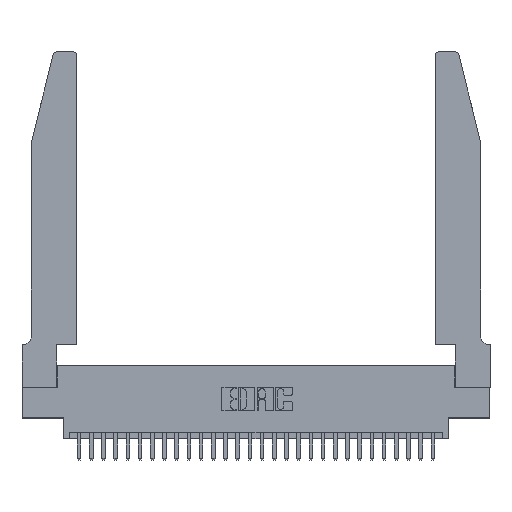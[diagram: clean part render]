
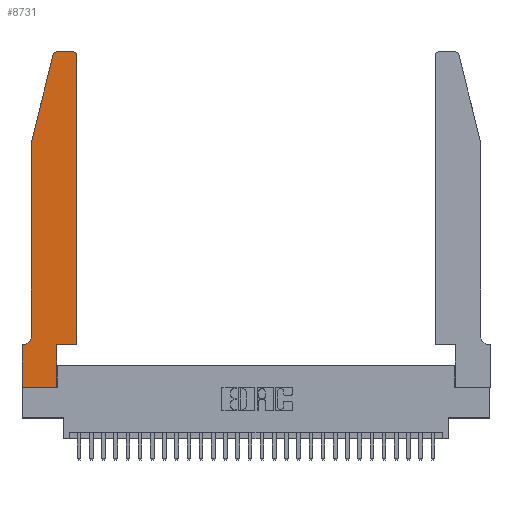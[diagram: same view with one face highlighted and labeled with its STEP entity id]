
A CAD part, top view. The second image highlights one B-rep face of the part: STEP entity #8731.
In plain terms, the highlighted planar face has unit normal (0, 0, 1).
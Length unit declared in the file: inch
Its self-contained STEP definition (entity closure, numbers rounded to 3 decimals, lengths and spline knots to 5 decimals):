
#400 = DIRECTION ( 'NONE',  ( 0., 1., 0. ) ) ;
#866 = VERTEX_POINT ( 'NONE', #1583 ) ;
#1382 = VERTEX_POINT ( 'NONE', #17906 ) ;
#1514 = CARTESIAN_POINT ( 'NONE',  ( 0.4505, 2.72, 0.37 ) ) ;
#1583 = CARTESIAN_POINT ( 'NONE',  ( 0., 0., 0.37 ) ) ;
#1839 = ORIENTED_EDGE ( 'NONE', *, *, #29687, .T. ) ;
#2173 = DIRECTION ( 'NONE',  ( -1., 0., 0. ) ) ;
#2347 = DIRECTION ( 'NONE',  ( 0., 0., 1. ) ) ;
#2519 = AXIS2_PLACEMENT_3D ( 'NONE', #6919, #2347, #13959 ) ;
#2740 = FACE_OUTER_BOUND ( 'NONE', #25307, .T. ) ;
#2749 = LINE ( 'NONE', #6839, #7132 ) ;
#3153 = DIRECTION ( 'NONE',  ( 1., 0., 0. ) ) ;
#3450 = VECTOR ( 'NONE', #23877, 39.37008 ) ;
#3625 = CARTESIAN_POINT ( 'NONE',  ( 0.0055, 0.42, 0.37 ) ) ;
#4006 = ORIENTED_EDGE ( 'NONE', *, *, #6376, .T. ) ;
#4008 = CARTESIAN_POINT ( 'NONE',  ( 0., 0., 0.37 ) ) ;
#4058 = EDGE_CURVE ( 'NONE', #866, #12160, #10639, .T. ) ;
#4547 = DIRECTION ( 'NONE',  ( 1., 0., 0. ) ) ;
#4774 = CARTESIAN_POINT ( 'NONE',  ( 0.4505, 0.35, 0.37 ) ) ;
#5276 = DIRECTION ( 'NONE',  ( 0., 0., 1. ) ) ;
#5450 = VECTOR ( 'NONE', #4547, 39.37008 ) ;
#5524 = ORIENTED_EDGE ( 'NONE', *, *, #20856, .T. ) ;
#5553 = CIRCLE ( 'NONE', #29650, 0.03 ) ;
#5949 = ORIENTED_EDGE ( 'NONE', *, *, #25968, .T. ) ;
#6006 = CIRCLE ( 'NONE', #2519, 0.03 ) ;
#6342 = DIRECTION ( 'NONE',  ( 0., -1., 0. ) ) ;
#6376 = EDGE_CURVE ( 'NONE', #15436, #26476, #27697, .T. ) ;
#6839 = CARTESIAN_POINT ( 'NONE',  ( 0.2605, 2.75, 0.37 ) ) ;
#6919 = CARTESIAN_POINT ( 'NONE',  ( 0.4205, 2.72, 0.37 ) ) ;
#7031 = CARTESIAN_POINT ( 'NONE',  ( 0.0755, 2., 0.37 ) ) ;
#7132 = VECTOR ( 'NONE', #2173, 39.37008 ) ;
#8119 = LINE ( 'NONE', #4008, #30010 ) ;
#8731 = ADVANCED_FACE ( 'NONE', ( #2740 ), #18936, .T. ) ;
#8822 = CARTESIAN_POINT ( 'NONE',  ( 0.2865, 0.35, 0.37 ) ) ;
#8891 = ORIENTED_EDGE ( 'NONE', *, *, #12074, .T. ) ;
#9336 = CARTESIAN_POINT ( 'NONE',  ( 0.0755, 2., 0.37 ) ) ;
#9590 = AXIS2_PLACEMENT_3D ( 'NONE', #3625, #29601, #19929 ) ;
#9605 = CARTESIAN_POINT ( 'NONE',  ( 0.2865, 0.35, 0.37 ) ) ;
#9674 = VERTEX_POINT ( 'NONE', #12147 ) ;
#10113 = VECTOR ( 'NONE', #14328, 39.37008 ) ;
#10639 = LINE ( 'NONE', #22815, #20156 ) ;
#11141 = DIRECTION ( 'NONE',  ( 1., 0., 0. ) ) ;
#11962 = VECTOR ( 'NONE', #400, 39.37008 ) ;
#12029 = EDGE_CURVE ( 'NONE', #24052, #18777, #6006, .T. ) ;
#12074 = EDGE_CURVE ( 'NONE', #20409, #1382, #23159, .T. ) ;
#12147 = CARTESIAN_POINT ( 'NONE',  ( 0.0055, 0.35, 0.37 ) ) ;
#12160 = VERTEX_POINT ( 'NONE', #24199 ) ;
#13611 = CARTESIAN_POINT ( 'NONE',  ( 0.284, 2.72, 0.37 ) ) ;
#13959 = DIRECTION ( 'NONE',  ( 1., 0., 0. ) ) ;
#14328 = DIRECTION ( 'NONE',  ( 0., 1., 0. ) ) ;
#14569 = CARTESIAN_POINT ( 'NONE',  ( 0., 0.35, 0.37 ) ) ;
#14769 = VECTOR ( 'NONE', #19627, 39.37008 ) ;
#14850 = CARTESIAN_POINT ( 'NONE',  ( 0.25487, 2.72718, 0.37 ) ) ;
#14970 = CIRCLE ( 'NONE', #9590, 0.07 ) ;
#15436 = VERTEX_POINT ( 'NONE', #8822 ) ;
#15890 = ORIENTED_EDGE ( 'NONE', *, *, #29609, .T. ) ;
#15898 = VERTEX_POINT ( 'NONE', #14850 ) ;
#16619 = LINE ( 'NONE', #28570, #3450 ) ;
#17529 = CARTESIAN_POINT ( 'NONE',  ( 0.284, 2.75, 0.37 ) ) ;
#17640 = DIRECTION ( 'NONE',  ( 1., 0., 0. ) ) ;
#17720 = ORIENTED_EDGE ( 'NONE', *, *, #4058, .T. ) ;
#17862 = VERTEX_POINT ( 'NONE', #28908 ) ;
#17906 = CARTESIAN_POINT ( 'NONE',  ( 0.0755, 0.42, 0.37 ) ) ;
#18518 = CARTESIAN_POINT ( 'NONE',  ( 0.4505, 0.35, 0.37 ) ) ;
#18777 = VERTEX_POINT ( 'NONE', #29629 ) ;
#18936 = PLANE ( 'NONE',  #28806 ) ;
#19627 = DIRECTION ( 'NONE',  ( 0., -1., 0. ) ) ;
#19929 = DIRECTION ( 'NONE',  ( -1., 0., 0. ) ) ;
#20156 = VECTOR ( 'NONE', #17640, 39.37008 ) ;
#20280 = CARTESIAN_POINT ( 'NONE',  ( 0.4505, 0.35, 0.37 ) ) ;
#20409 = VERTEX_POINT ( 'NONE', #21450 ) ;
#20549 = DIRECTION ( 'NONE',  ( 0., 0., 1. ) ) ;
#20760 = ORIENTED_EDGE ( 'NONE', *, *, #12029, .T. ) ;
#20856 = EDGE_CURVE ( 'NONE', #18777, #29926, #2749, .T. ) ;
#21446 = LINE ( 'NONE', #7031, #22934 ) ;
#21450 = CARTESIAN_POINT ( 'NONE',  ( 0.0755, 2., 0.37 ) ) ;
#21669 = ORIENTED_EDGE ( 'NONE', *, *, #24175, .T. ) ;
#21789 = EDGE_CURVE ( 'NONE', #9674, #17862, #16619, .T. ) ;
#22815 = CARTESIAN_POINT ( 'NONE',  ( 0., 0., 0.37 ) ) ;
#22934 = VECTOR ( 'NONE', #28540, 39.37008 ) ;
#23003 = EDGE_CURVE ( 'NONE', #12160, #15436, #29819, .T. ) ;
#23159 = LINE ( 'NONE', #9336, #14769 ) ;
#23877 = DIRECTION ( 'NONE',  ( -1., 0., 0. ) ) ;
#24052 = VERTEX_POINT ( 'NONE', #1514 ) ;
#24175 = EDGE_CURVE ( 'NONE', #29926, #15898, #5553, .T. ) ;
#24199 = CARTESIAN_POINT ( 'NONE',  ( 0.2865, 0., 0.37 ) ) ;
#24354 = LINE ( 'NONE', #4774, #11962 ) ;
#25307 = EDGE_LOOP ( 'NONE', ( #5524, #21669, #1839, #8891, #27324, #28765, #5949, #17720, #26586, #4006, #15890, #20760 ) ) ;
#25968 = EDGE_CURVE ( 'NONE', #17862, #866, #8119, .T. ) ;
#26476 = VERTEX_POINT ( 'NONE', #20280 ) ;
#26586 = ORIENTED_EDGE ( 'NONE', *, *, #23003, .T. ) ;
#27324 = ORIENTED_EDGE ( 'NONE', *, *, #28725, .T. ) ;
#27697 = LINE ( 'NONE', #18518, #5450 ) ;
#28540 = DIRECTION ( 'NONE',  ( -0.239, -0.971, 0. ) ) ;
#28570 = CARTESIAN_POINT ( 'NONE',  ( 0.0755, 0.35, 0.37 ) ) ;
#28725 = EDGE_CURVE ( 'NONE', #1382, #9674, #14970, .T. ) ;
#28765 = ORIENTED_EDGE ( 'NONE', *, *, #21789, .T. ) ;
#28806 = AXIS2_PLACEMENT_3D ( 'NONE', #14569, #5276, #3153 ) ;
#28908 = CARTESIAN_POINT ( 'NONE',  ( 0., 0.35, 0.37 ) ) ;
#29601 = DIRECTION ( 'NONE',  ( 0., 0., -1. ) ) ;
#29609 = EDGE_CURVE ( 'NONE', #26476, #24052, #24354, .T. ) ;
#29629 = CARTESIAN_POINT ( 'NONE',  ( 0.4205, 2.75, 0.37 ) ) ;
#29650 = AXIS2_PLACEMENT_3D ( 'NONE', #13611, #20549, #11141 ) ;
#29687 = EDGE_CURVE ( 'NONE', #15898, #20409, #21446, .T. ) ;
#29819 = LINE ( 'NONE', #9605, #10113 ) ;
#29926 = VERTEX_POINT ( 'NONE', #17529 ) ;
#30010 = VECTOR ( 'NONE', #6342, 39.37008 ) ;
